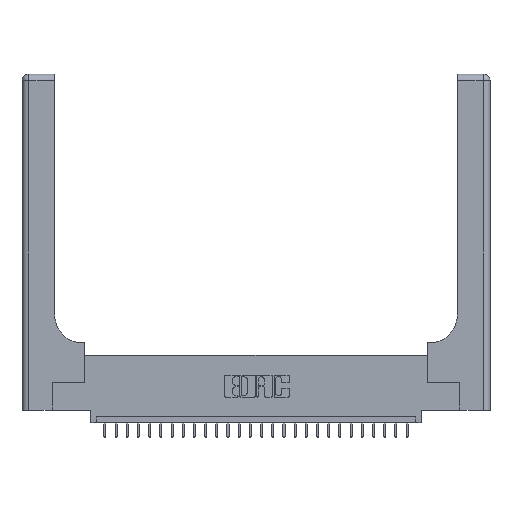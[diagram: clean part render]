
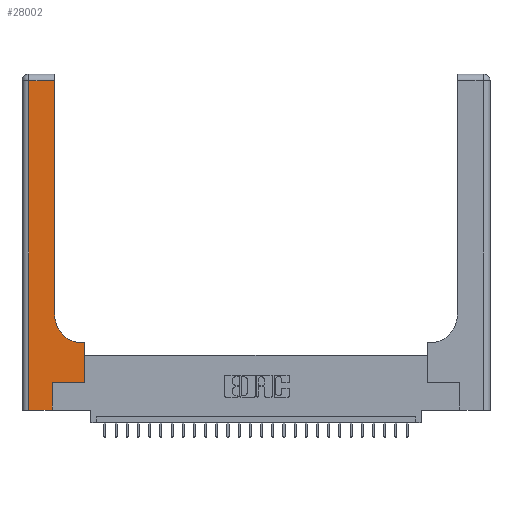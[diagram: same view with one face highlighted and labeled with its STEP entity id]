
A CAD part, top view. The second image highlights one B-rep face of the part: STEP entity #28002.
In plain terms, the highlighted planar face has unit normal (0, 0, 1).
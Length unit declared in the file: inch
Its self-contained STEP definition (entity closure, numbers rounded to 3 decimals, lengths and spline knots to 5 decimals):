
#97 = LINE ( 'NONE', #19299, #17401 ) ;
#280 = LINE ( 'NONE', #12075, #13198 ) ;
#884 = LINE ( 'NONE', #11751, #2566 ) ;
#1076 = AXIS2_PLACEMENT_3D ( 'NONE', #18287, #7375, #1087 ) ;
#1087 = DIRECTION ( 'NONE',  ( -1., 0., 0. ) ) ;
#1541 = EDGE_CURVE ( 'NONE', #23424, #28048, #280, .T. ) ;
#1988 = VERTEX_POINT ( 'NONE', #22591 ) ;
#2566 = VECTOR ( 'NONE', #9596, 39.37008 ) ;
#3294 = ORIENTED_EDGE ( 'NONE', *, *, #27556, .T. ) ;
#3705 = VECTOR ( 'NONE', #28026, 39.37008 ) ;
#3819 = CARTESIAN_POINT ( 'NONE',  ( 0.269, 0., 0.37 ) ) ;
#4558 = ORIENTED_EDGE ( 'NONE', *, *, #22366, .T. ) ;
#4726 = VECTOR ( 'NONE', #16163, 39.37008 ) ;
#5267 = CARTESIAN_POINT ( 'NONE',  ( 0.269, 0., 0.37 ) ) ;
#5274 = DIRECTION ( 'NONE',  ( -1., 0., 0. ) ) ;
#6028 = LINE ( 'NONE', #14914, #3705 ) ;
#6516 = CARTESIAN_POINT ( 'NONE',  ( 0.2915, 2.94, 0.37 ) ) ;
#7375 = DIRECTION ( 'NONE',  ( 0., 0., -1. ) ) ;
#7436 = CARTESIAN_POINT ( 'NONE',  ( 0.06, 3., 0.37 ) ) ;
#7722 = DIRECTION ( 'NONE',  ( 0., -1., 0. ) ) ;
#8773 = ORIENTED_EDGE ( 'NONE', *, *, #25239, .T. ) ;
#8960 = CARTESIAN_POINT ( 'NONE',  ( 0.5415, 0.85, 0.37 ) ) ;
#9531 = PLANE ( 'NONE',  #1076 ) ;
#9596 = DIRECTION ( 'NONE',  ( 0., 1., 0. ) ) ;
#9850 = CARTESIAN_POINT ( 'NONE',  ( 0.2915, 0.6, 0.37 ) ) ;
#10765 = CARTESIAN_POINT ( 'NONE',  ( 0.5585, 0.6, 0.37 ) ) ;
#10948 = CARTESIAN_POINT ( 'NONE',  ( 0.5585, 0.25, 0.37 ) ) ;
#10966 = VECTOR ( 'NONE', #7722, 39.37008 ) ;
#11751 = CARTESIAN_POINT ( 'NONE',  ( 0.5585, 0.25, 0.37 ) ) ;
#12075 = CARTESIAN_POINT ( 'NONE',  ( 0., 0., 0.37 ) ) ;
#12087 = VERTEX_POINT ( 'NONE', #10948 ) ;
#12465 = CARTESIAN_POINT ( 'NONE',  ( 0.269, 0.25, 0.37 ) ) ;
#12930 = VERTEX_POINT ( 'NONE', #12465 ) ;
#12973 = ORIENTED_EDGE ( 'NONE', *, *, #17547, .T. ) ;
#13198 = VECTOR ( 'NONE', #27478, 39.37008 ) ;
#14247 = FACE_OUTER_BOUND ( 'NONE', #27074, .T. ) ;
#14790 = CARTESIAN_POINT ( 'NONE',  ( 0.06, 2.94, 0.37 ) ) ;
#14914 = CARTESIAN_POINT ( 'NONE',  ( 0.269, 0.25, 0.37 ) ) ;
#15572 = DIRECTION ( 'NONE',  ( 1., 0., 0. ) ) ;
#15783 = ORIENTED_EDGE ( 'NONE', *, *, #18040, .T. ) ;
#16163 = DIRECTION ( 'NONE',  ( 0., 1., 0. ) ) ;
#17019 = ORIENTED_EDGE ( 'NONE', *, *, #25233, .T. ) ;
#17169 = DIRECTION ( 'NONE',  ( 0., 1., 0. ) ) ;
#17217 = ORIENTED_EDGE ( 'NONE', *, *, #26731, .T. ) ;
#17401 = VECTOR ( 'NONE', #23449, 39.37008 ) ;
#17547 = EDGE_CURVE ( 'NONE', #19616, #23424, #18076, .T. ) ;
#18040 = EDGE_CURVE ( 'NONE', #18116, #19616, #97, .T. ) ;
#18076 = LINE ( 'NONE', #7436, #10966 ) ;
#18116 = VERTEX_POINT ( 'NONE', #6516 ) ;
#18287 = CARTESIAN_POINT ( 'NONE',  ( 0., 3., 0.37 ) ) ;
#18305 = LINE ( 'NONE', #27110, #4726 ) ;
#19299 = CARTESIAN_POINT ( 'NONE',  ( 0., 2.94, 0.37 ) ) ;
#19522 = CARTESIAN_POINT ( 'NONE',  ( 0.06, 0., 0.37 ) ) ;
#19616 = VERTEX_POINT ( 'NONE', #14790 ) ;
#20033 = DIRECTION ( 'NONE',  ( 0., 0., -1. ) ) ;
#20174 = EDGE_CURVE ( 'NONE', #12930, #12087, #6028, .T. ) ;
#20687 = VECTOR ( 'NONE', #5274, 39.37008 ) ;
#20697 = ORIENTED_EDGE ( 'NONE', *, *, #20174, .T. ) ;
#20736 = LINE ( 'NONE', #9850, #20687 ) ;
#21263 = CIRCLE ( 'NONE', #24045, 0.25 ) ;
#21543 = CARTESIAN_POINT ( 'NONE',  ( 0.2915, 0.85, 0.37 ) ) ;
#22366 = EDGE_CURVE ( 'NONE', #24611, #1988, #20736, .T. ) ;
#22591 = CARTESIAN_POINT ( 'NONE',  ( 0.5415, 0.6, 0.37 ) ) ;
#23051 = ORIENTED_EDGE ( 'NONE', *, *, #1541, .T. ) ;
#23424 = VERTEX_POINT ( 'NONE', #19522 ) ;
#23449 = DIRECTION ( 'NONE',  ( -1., 0., 0. ) ) ;
#24045 = AXIS2_PLACEMENT_3D ( 'NONE', #8960, #20033, #15572 ) ;
#24611 = VERTEX_POINT ( 'NONE', #10765 ) ;
#24926 = LINE ( 'NONE', #5267, #25820 ) ;
#25233 = EDGE_CURVE ( 'NONE', #27488, #18116, #18305, .T. ) ;
#25239 = EDGE_CURVE ( 'NONE', #28048, #12930, #24926, .T. ) ;
#25820 = VECTOR ( 'NONE', #17169, 39.37008 ) ;
#26731 = EDGE_CURVE ( 'NONE', #1988, #27488, #21263, .T. ) ;
#27074 = EDGE_LOOP ( 'NONE', ( #17019, #15783, #12973, #23051, #8773, #20697, #3294, #4558, #17217 ) ) ;
#27110 = CARTESIAN_POINT ( 'NONE',  ( 0.2915, 3., 0.37 ) ) ;
#27478 = DIRECTION ( 'NONE',  ( 1., 0., 0. ) ) ;
#27488 = VERTEX_POINT ( 'NONE', #21543 ) ;
#27556 = EDGE_CURVE ( 'NONE', #12087, #24611, #884, .T. ) ;
#28002 = ADVANCED_FACE ( 'NONE', ( #14247 ), #9531, .F. ) ;
#28026 = DIRECTION ( 'NONE',  ( 1., 0., 0. ) ) ;
#28048 = VERTEX_POINT ( 'NONE', #3819 ) ;
